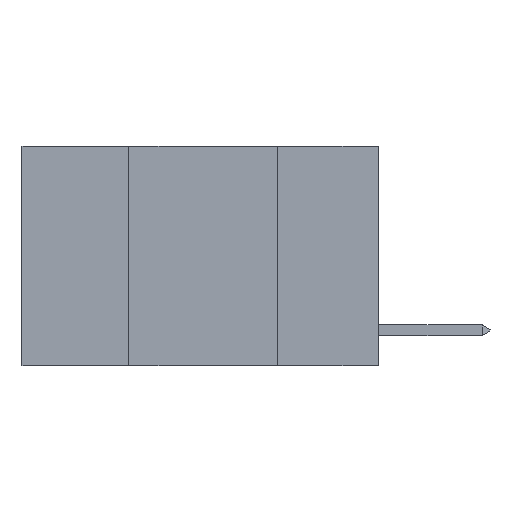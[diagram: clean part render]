
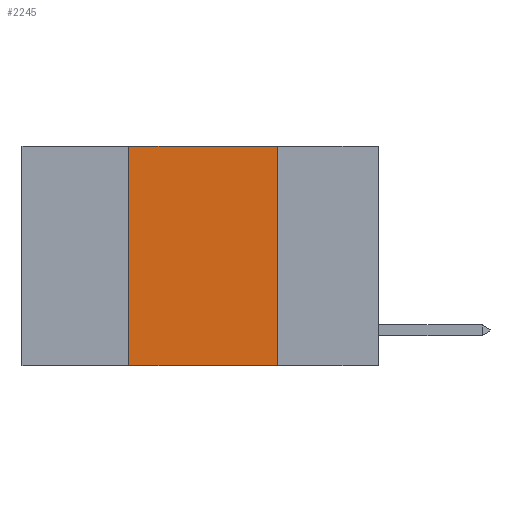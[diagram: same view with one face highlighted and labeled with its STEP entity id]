
A CAD part, left-side view. The second image highlights one B-rep face of the part: STEP entity #2245.
In plain terms, the highlighted planar face has unit normal (-1, 0, 0).
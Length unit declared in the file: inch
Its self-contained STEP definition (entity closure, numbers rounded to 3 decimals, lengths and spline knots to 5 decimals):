
#413 = DIRECTION ( 'NONE',  ( 0., 0., -1. ) ) ;
#1726 = AXIS2_PLACEMENT_3D ( 'NONE', #11930, #11711, #11651 ) ;
#1791 = CARTESIAN_POINT ( 'NONE',  ( 0., 0.17, -0.37 ) ) ;
#2245 = ADVANCED_FACE ( 'NONE', ( #13739 ), #11771, .F. ) ;
#2551 = VERTEX_POINT ( 'NONE', #7833 ) ;
#2668 = DIRECTION ( 'NONE',  ( 0., -1., 0. ) ) ;
#3566 = LINE ( 'NONE', #9511, #16311 ) ;
#3823 = CARTESIAN_POINT ( 'NONE',  ( 0., 0.6, -0.37 ) ) ;
#4097 = ORIENTED_EDGE ( 'NONE', *, *, #6881, .F. ) ;
#4174 = VECTOR ( 'NONE', #2668, 39.37008 ) ;
#4271 = CARTESIAN_POINT ( 'NONE',  ( 0., 0.17, 0. ) ) ;
#4387 = CARTESIAN_POINT ( 'NONE',  ( 0., 0.42, 0. ) ) ;
#6449 = EDGE_LOOP ( 'NONE', ( #13657, #12193, #4097, #8904 ) ) ;
#6551 = EDGE_CURVE ( 'NONE', #12957, #8722, #7986, .T. ) ;
#6881 = EDGE_CURVE ( 'NONE', #12957, #12545, #3566, .T. ) ;
#7833 = CARTESIAN_POINT ( 'NONE',  ( 0., 0.17, 0. ) ) ;
#7986 = LINE ( 'NONE', #3823, #14329 ) ;
#8722 = VERTEX_POINT ( 'NONE', #1791 ) ;
#8904 = ORIENTED_EDGE ( 'NONE', *, *, #6551, .T. ) ;
#9511 = CARTESIAN_POINT ( 'NONE',  ( 0., 0.42, 0. ) ) ;
#10809 = DIRECTION ( 'NONE',  ( 0., 0., 1. ) ) ;
#11588 = CARTESIAN_POINT ( 'NONE',  ( 0., 0.6, 0. ) ) ;
#11651 = DIRECTION ( 'NONE',  ( 0., 0., -1. ) ) ;
#11711 = DIRECTION ( 'NONE',  ( 1., 0., 0. ) ) ;
#11771 = PLANE ( 'NONE',  #1726 ) ;
#11821 = CARTESIAN_POINT ( 'NONE',  ( 0., 0.42, -0.37 ) ) ;
#11930 = CARTESIAN_POINT ( 'NONE',  ( 0., 0.6, 0. ) ) ;
#12072 = VECTOR ( 'NONE', #413, 39.37008 ) ;
#12193 = ORIENTED_EDGE ( 'NONE', *, *, #13511, .F. ) ;
#12545 = VERTEX_POINT ( 'NONE', #4387 ) ;
#12957 = VERTEX_POINT ( 'NONE', #11821 ) ;
#13511 = EDGE_CURVE ( 'NONE', #12545, #2551, #14134, .T. ) ;
#13657 = ORIENTED_EDGE ( 'NONE', *, *, #15917, .F. ) ;
#13739 = FACE_OUTER_BOUND ( 'NONE', #6449, .T. ) ;
#14010 = DIRECTION ( 'NONE',  ( 0., -1., 0. ) ) ;
#14134 = LINE ( 'NONE', #11588, #4174 ) ;
#14329 = VECTOR ( 'NONE', #14010, 39.37008 ) ;
#15443 = LINE ( 'NONE', #4271, #12072 ) ;
#15917 = EDGE_CURVE ( 'NONE', #2551, #8722, #15443, .T. ) ;
#16311 = VECTOR ( 'NONE', #10809, 39.37008 ) ;
